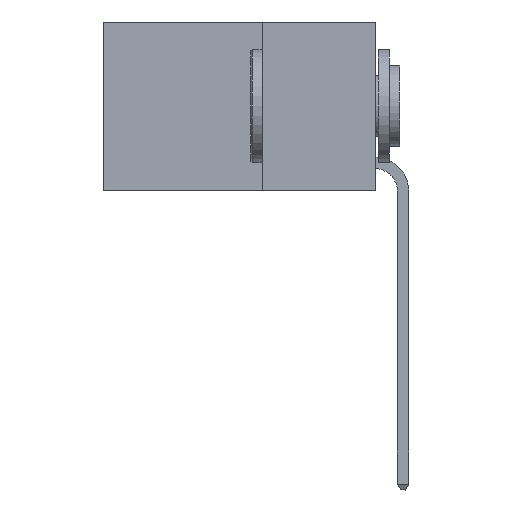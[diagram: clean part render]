
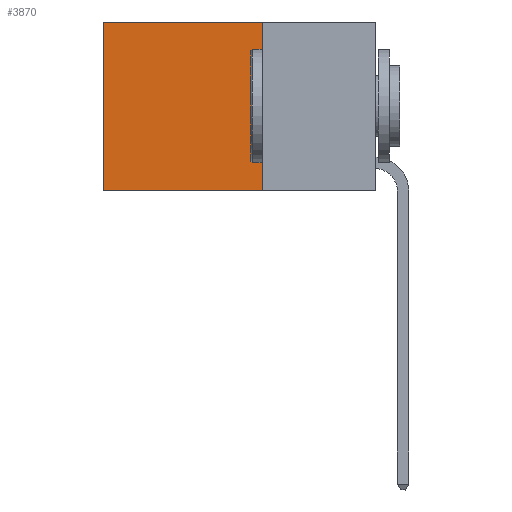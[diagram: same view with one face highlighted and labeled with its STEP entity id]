
A CAD part, left-side view. The second image highlights one B-rep face of the part: STEP entity #3870.
In plain terms, the highlighted planar face has unit normal (-1, 0, 0).
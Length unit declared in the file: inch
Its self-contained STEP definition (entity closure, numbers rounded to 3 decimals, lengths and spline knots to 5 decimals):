
#508 = CARTESIAN_POINT ( 'NONE',  ( 0.2625, 0.25, 0. ) ) ;
#1613 = AXIS2_PLACEMENT_3D ( 'NONE', #7768, #17373, #9164 ) ;
#1663 = VECTOR ( 'NONE', #12523, 39.37008 ) ;
#2117 = ORIENTED_EDGE ( 'NONE', *, *, #16906, .F. ) ;
#2512 = ORIENTED_EDGE ( 'NONE', *, *, #4786, .T. ) ;
#2738 = VERTEX_POINT ( 'NONE', #9504 ) ;
#3115 = VECTOR ( 'NONE', #4795, 39.37008 ) ;
#3870 = ADVANCED_FACE ( 'NONE', ( #9216 ), #15999, .F. ) ;
#4082 = CARTESIAN_POINT ( 'NONE',  ( 0.2625, 0.25, 0. ) ) ;
#4592 = LINE ( 'NONE', #11150, #1663 ) ;
#4786 = EDGE_CURVE ( 'NONE', #15076, #2738, #4592, .T. ) ;
#4795 = DIRECTION ( 'NONE',  ( 0., 1., 0. ) ) ;
#6905 = DIRECTION ( 'NONE',  ( 0., 1., 0. ) ) ;
#7103 = VECTOR ( 'NONE', #6905, 39.37008 ) ;
#7768 = CARTESIAN_POINT ( 'NONE',  ( 0.2625, 0.25, 0. ) ) ;
#7800 = CARTESIAN_POINT ( 'NONE',  ( 0.2625, 0.25, -0.37 ) ) ;
#7889 = LINE ( 'NONE', #17173, #15215 ) ;
#8795 = ORIENTED_EDGE ( 'NONE', *, *, #15148, .T. ) ;
#8871 = EDGE_LOOP ( 'NONE', ( #2512, #2117, #12449, #8795 ) ) ;
#8957 = DIRECTION ( 'NONE',  ( 0., 0., -1. ) ) ;
#9164 = DIRECTION ( 'NONE',  ( 0., 0., -1. ) ) ;
#9216 = FACE_OUTER_BOUND ( 'NONE', #8871, .T. ) ;
#9504 = CARTESIAN_POINT ( 'NONE',  ( 0.2625, 0.6, -0.37 ) ) ;
#10057 = VERTEX_POINT ( 'NONE', #7800 ) ;
#10278 = CARTESIAN_POINT ( 'NONE',  ( 0.2625, 0.25, -0.37 ) ) ;
#11150 = CARTESIAN_POINT ( 'NONE',  ( 0.2625, 0.6, 0. ) ) ;
#11262 = EDGE_CURVE ( 'NONE', #16922, #10057, #7889, .T. ) ;
#12193 = LINE ( 'NONE', #4082, #7103 ) ;
#12449 = ORIENTED_EDGE ( 'NONE', *, *, #11262, .F. ) ;
#12523 = DIRECTION ( 'NONE',  ( 0., 0., -1. ) ) ;
#13612 = CARTESIAN_POINT ( 'NONE',  ( 0.2625, 0.6, 0. ) ) ;
#15076 = VERTEX_POINT ( 'NONE', #13612 ) ;
#15148 = EDGE_CURVE ( 'NONE', #16922, #15076, #12193, .T. ) ;
#15215 = VECTOR ( 'NONE', #8957, 39.37008 ) ;
#15999 = PLANE ( 'NONE',  #1613 ) ;
#16906 = EDGE_CURVE ( 'NONE', #10057, #2738, #17406, .T. ) ;
#16922 = VERTEX_POINT ( 'NONE', #508 ) ;
#17173 = CARTESIAN_POINT ( 'NONE',  ( 0.2625, 0.25, 0. ) ) ;
#17373 = DIRECTION ( 'NONE',  ( 1., 0., 0. ) ) ;
#17406 = LINE ( 'NONE', #10278, #3115 ) ;
